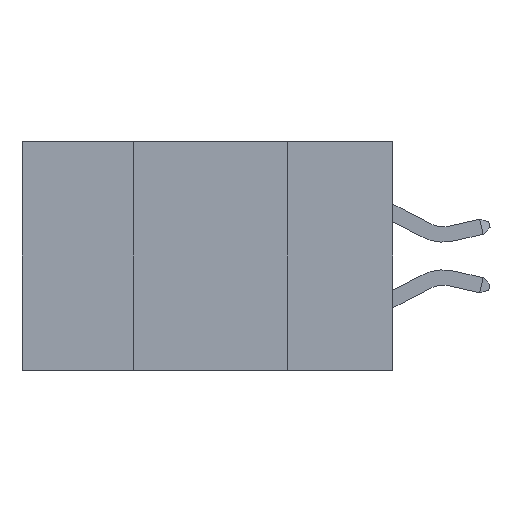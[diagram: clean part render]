
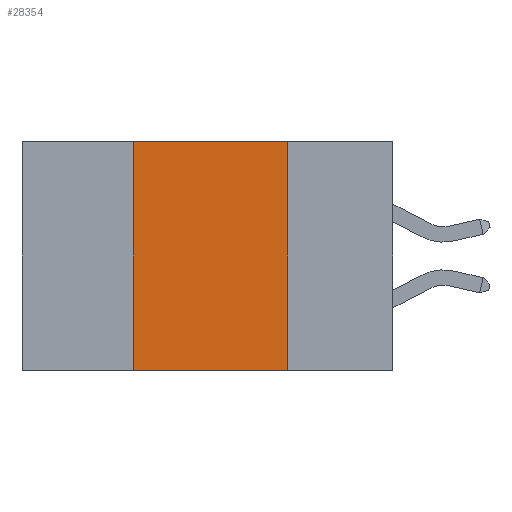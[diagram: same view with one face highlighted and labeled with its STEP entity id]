
A CAD part, left-side view. The second image highlights one B-rep face of the part: STEP entity #28354.
In plain terms, the highlighted planar face has unit normal (-1, 0, 0).
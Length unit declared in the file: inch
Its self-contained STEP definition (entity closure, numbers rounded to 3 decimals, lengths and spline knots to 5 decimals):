
#159 = EDGE_CURVE ( 'NONE', #6130, #10411, #8390, .T. ) ;
#1366 = VECTOR ( 'NONE', #2018, 39.37008 ) ;
#1491 = VERTEX_POINT ( 'NONE', #12929 ) ;
#1946 = DIRECTION ( 'NONE',  ( 0., 0., -1. ) ) ;
#2018 = DIRECTION ( 'NONE',  ( 0., 0., -1. ) ) ;
#5296 = LINE ( 'NONE', #19204, #21058 ) ;
#6053 = DIRECTION ( 'NONE',  ( 1., 0., 0. ) ) ;
#6130 = VERTEX_POINT ( 'NONE', #9797 ) ;
#6567 = EDGE_CURVE ( 'NONE', #1491, #25212, #21398, .T. ) ;
#7323 = CARTESIAN_POINT ( 'NONE',  ( 0., 0.17, -0.37 ) ) ;
#8390 = LINE ( 'NONE', #24698, #25740 ) ;
#9797 = CARTESIAN_POINT ( 'NONE',  ( 0., 0.42, 0. ) ) ;
#10411 = VERTEX_POINT ( 'NONE', #20259 ) ;
#10910 = ORIENTED_EDGE ( 'NONE', *, *, #15194, .F. ) ;
#12617 = EDGE_LOOP ( 'NONE', ( #14514, #12688, #10910, #23843 ) ) ;
#12688 = ORIENTED_EDGE ( 'NONE', *, *, #159, .F. ) ;
#12764 = DIRECTION ( 'NONE',  ( 0., -1., 0. ) ) ;
#12929 = CARTESIAN_POINT ( 'NONE',  ( 0., 0.42, -0.37 ) ) ;
#14514 = ORIENTED_EDGE ( 'NONE', *, *, #27966, .F. ) ;
#15194 = EDGE_CURVE ( 'NONE', #1491, #6130, #5296, .T. ) ;
#15275 = CARTESIAN_POINT ( 'NONE',  ( 0., 0.6, 0. ) ) ;
#15935 = LINE ( 'NONE', #25152, #1366 ) ;
#19204 = CARTESIAN_POINT ( 'NONE',  ( 0., 0.42, 0. ) ) ;
#19244 = AXIS2_PLACEMENT_3D ( 'NONE', #15275, #6053, #1946 ) ;
#20259 = CARTESIAN_POINT ( 'NONE',  ( 0., 0.17, 0. ) ) ;
#21058 = VECTOR ( 'NONE', #24320, 39.37008 ) ;
#21398 = LINE ( 'NONE', #28355, #23670 ) ;
#23670 = VECTOR ( 'NONE', #26089, 39.37008 ) ;
#23843 = ORIENTED_EDGE ( 'NONE', *, *, #6567, .T. ) ;
#24320 = DIRECTION ( 'NONE',  ( 0., 0., 1. ) ) ;
#24698 = CARTESIAN_POINT ( 'NONE',  ( 0., 0.6, 0. ) ) ;
#24944 = PLANE ( 'NONE',  #19244 ) ;
#25152 = CARTESIAN_POINT ( 'NONE',  ( 0., 0.17, 0. ) ) ;
#25212 = VERTEX_POINT ( 'NONE', #7323 ) ;
#25740 = VECTOR ( 'NONE', #12764, 39.37008 ) ;
#26089 = DIRECTION ( 'NONE',  ( 0., -1., 0. ) ) ;
#26755 = FACE_OUTER_BOUND ( 'NONE', #12617, .T. ) ;
#27966 = EDGE_CURVE ( 'NONE', #10411, #25212, #15935, .T. ) ;
#28354 = ADVANCED_FACE ( 'NONE', ( #26755 ), #24944, .F. ) ;
#28355 = CARTESIAN_POINT ( 'NONE',  ( 0., 0.6, -0.37 ) ) ;
